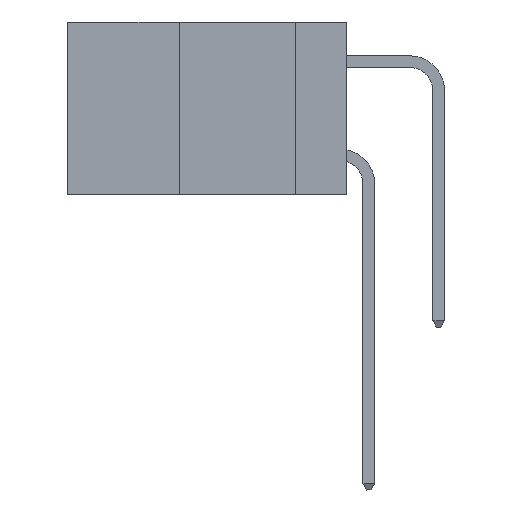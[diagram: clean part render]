
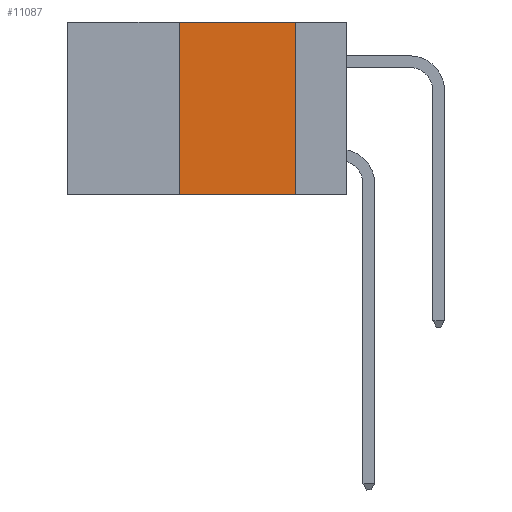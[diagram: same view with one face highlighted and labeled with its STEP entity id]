
A CAD part, left-side view. The second image highlights one B-rep face of the part: STEP entity #11087.
In plain terms, the highlighted planar face has unit normal (-1, 0, 0).
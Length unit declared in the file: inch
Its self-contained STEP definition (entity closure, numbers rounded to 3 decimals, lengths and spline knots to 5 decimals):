
#374 = DIRECTION ( 'NONE',  ( 0., 0., -1. ) ) ;
#489 = DIRECTION ( 'NONE',  ( 0., 0., 1. ) ) ;
#587 = CARTESIAN_POINT ( 'NONE',  ( 0., 0.6, 0. ) ) ;
#1893 = LINE ( 'NONE', #11879, #11449 ) ;
#2329 = EDGE_CURVE ( 'NONE', #6851, #8136, #18795, .T. ) ;
#4326 = DIRECTION ( 'NONE',  ( 0., -1., 0. ) ) ;
#4592 = LINE ( 'NONE', #22957, #14053 ) ;
#5187 = ORIENTED_EDGE ( 'NONE', *, *, #2329, .T. ) ;
#5413 = EDGE_CURVE ( 'NONE', #8674, #9574, #17239, .T. ) ;
#6245 = CARTESIAN_POINT ( 'NONE',  ( 0., 0.11, 0. ) ) ;
#6851 = VERTEX_POINT ( 'NONE', #13189 ) ;
#8136 = VERTEX_POINT ( 'NONE', #22342 ) ;
#8674 = VERTEX_POINT ( 'NONE', #11288 ) ;
#8962 = CARTESIAN_POINT ( 'NONE',  ( 0., 0.6, 0. ) ) ;
#9574 = VERTEX_POINT ( 'NONE', #6245 ) ;
#10767 = EDGE_LOOP ( 'NONE', ( #20608, #10829, #12672, #5187 ) ) ;
#10829 = ORIENTED_EDGE ( 'NONE', *, *, #5413, .F. ) ;
#10864 = DIRECTION ( 'NONE',  ( 0., 0., -1. ) ) ;
#11087 = ADVANCED_FACE ( 'NONE', ( #24180 ), #20087, .F. ) ;
#11288 = CARTESIAN_POINT ( 'NONE',  ( 0., 0.36, 0. ) ) ;
#11449 = VECTOR ( 'NONE', #374, 39.37008 ) ;
#11694 = VECTOR ( 'NONE', #17626, 39.37008 ) ;
#11879 = CARTESIAN_POINT ( 'NONE',  ( 0., 0.11, 0. ) ) ;
#12672 = ORIENTED_EDGE ( 'NONE', *, *, #20413, .F. ) ;
#13189 = CARTESIAN_POINT ( 'NONE',  ( 0., 0.36, -0.37 ) ) ;
#13929 = VECTOR ( 'NONE', #4326, 39.37008 ) ;
#14053 = VECTOR ( 'NONE', #489, 39.37008 ) ;
#14260 = AXIS2_PLACEMENT_3D ( 'NONE', #8962, #21891, #10864 ) ;
#15549 = EDGE_CURVE ( 'NONE', #9574, #8136, #1893, .T. ) ;
#17239 = LINE ( 'NONE', #587, #11694 ) ;
#17626 = DIRECTION ( 'NONE',  ( 0., -1., 0. ) ) ;
#18795 = LINE ( 'NONE', #22258, #13929 ) ;
#20087 = PLANE ( 'NONE',  #14260 ) ;
#20413 = EDGE_CURVE ( 'NONE', #6851, #8674, #4592, .T. ) ;
#20608 = ORIENTED_EDGE ( 'NONE', *, *, #15549, .F. ) ;
#21891 = DIRECTION ( 'NONE',  ( 1., 0., 0. ) ) ;
#22258 = CARTESIAN_POINT ( 'NONE',  ( 0., 0.6, -0.37 ) ) ;
#22342 = CARTESIAN_POINT ( 'NONE',  ( 0., 0.11, -0.37 ) ) ;
#22957 = CARTESIAN_POINT ( 'NONE',  ( 0., 0.36, 0. ) ) ;
#24180 = FACE_OUTER_BOUND ( 'NONE', #10767, .T. ) ;
